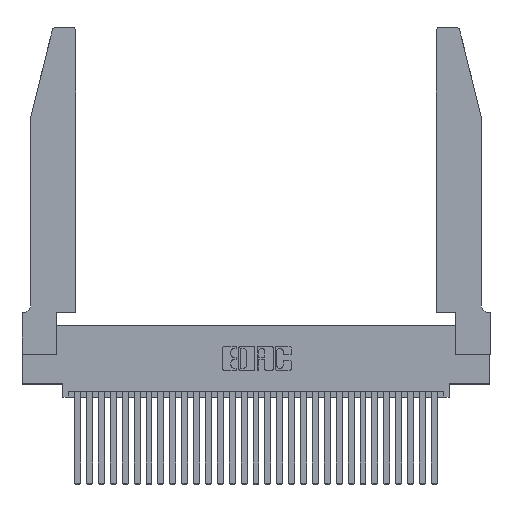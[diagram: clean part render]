
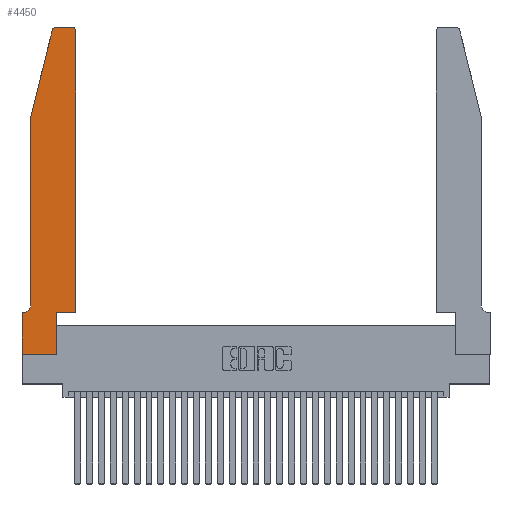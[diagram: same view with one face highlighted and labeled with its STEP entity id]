
A CAD part, top view. The second image highlights one B-rep face of the part: STEP entity #4450.
In plain terms, the highlighted planar face has unit normal (0, 0, 1).
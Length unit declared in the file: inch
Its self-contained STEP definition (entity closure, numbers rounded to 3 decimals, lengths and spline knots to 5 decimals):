
#511 = ORIENTED_EDGE ( 'NONE', *, *, #5564, .T. ) ;
#609 = LINE ( 'NONE', #2005, #8387 ) ;
#863 = VERTEX_POINT ( 'NONE', #15169 ) ;
#949 = VERTEX_POINT ( 'NONE', #22294 ) ;
#1247 = DIRECTION ( 'NONE',  ( 0., 1., 0. ) ) ;
#1689 = EDGE_CURVE ( 'NONE', #27433, #24652, #21861, .T. ) ;
#1990 = VECTOR ( 'NONE', #19626, 39.37008 ) ;
#2004 = ORIENTED_EDGE ( 'NONE', *, *, #20247, .T. ) ;
#2005 = CARTESIAN_POINT ( 'NONE',  ( 0., 0., 0.37 ) ) ;
#2236 = DIRECTION ( 'NONE',  ( 0., 0., -1. ) ) ;
#2530 = EDGE_LOOP ( 'NONE', ( #2004, #16556, #6188, #18421, #3329, #511, #29749, #9568, #21064, #11700, #13305, #5034 ) ) ;
#2979 = CIRCLE ( 'NONE', #29999, 0.03 ) ;
#3178 = LINE ( 'NONE', #10219, #20164 ) ;
#3296 = EDGE_CURVE ( 'NONE', #24652, #29688, #6993, .T. ) ;
#3329 = ORIENTED_EDGE ( 'NONE', *, *, #3296, .T. ) ;
#3477 = CARTESIAN_POINT ( 'NONE',  ( 0.4505, 0.35, 0.37 ) ) ;
#3782 = CARTESIAN_POINT ( 'NONE',  ( 0.284, 2.72, 0.37 ) ) ;
#4260 = CIRCLE ( 'NONE', #22508, 0.03 ) ;
#4450 = ADVANCED_FACE ( 'NONE', ( #7316 ), #19434, .T. ) ;
#4697 = CARTESIAN_POINT ( 'NONE',  ( 0., 0.35, 0.37 ) ) ;
#5034 = ORIENTED_EDGE ( 'NONE', *, *, #11345, .T. ) ;
#5291 = CARTESIAN_POINT ( 'NONE',  ( 0., 0.35, 0.37 ) ) ;
#5395 = CARTESIAN_POINT ( 'NONE',  ( 0.4505, 0.35, 0.37 ) ) ;
#5413 = EDGE_CURVE ( 'NONE', #16458, #863, #609, .T. ) ;
#5564 = EDGE_CURVE ( 'NONE', #29688, #20118, #5778, .T. ) ;
#5778 = LINE ( 'NONE', #12464, #22053 ) ;
#5947 = VERTEX_POINT ( 'NONE', #18750 ) ;
#6188 = ORIENTED_EDGE ( 'NONE', *, *, #13436, .T. ) ;
#6993 = CIRCLE ( 'NONE', #27061, 0.07 ) ;
#7275 = CARTESIAN_POINT ( 'NONE',  ( 0.0755, 2., 0.37 ) ) ;
#7316 = FACE_OUTER_BOUND ( 'NONE', #2530, .T. ) ;
#7475 = VECTOR ( 'NONE', #29697, 39.37008 ) ;
#7598 = CARTESIAN_POINT ( 'NONE',  ( 0.4505, 0.35, 0.37 ) ) ;
#7795 = CARTESIAN_POINT ( 'NONE',  ( 0.2865, 0.35, 0.37 ) ) ;
#8081 = DIRECTION ( 'NONE',  ( 1., 0., 0. ) ) ;
#8289 = CARTESIAN_POINT ( 'NONE',  ( 0.0755, 0.42, 0.37 ) ) ;
#8387 = VECTOR ( 'NONE', #18550, 39.37008 ) ;
#9568 = ORIENTED_EDGE ( 'NONE', *, *, #5413, .T. ) ;
#9693 = VERTEX_POINT ( 'NONE', #22281 ) ;
#10219 = CARTESIAN_POINT ( 'NONE',  ( 0., 0., 0.37 ) ) ;
#10857 = VECTOR ( 'NONE', #1247, 39.37008 ) ;
#11345 = EDGE_CURVE ( 'NONE', #26692, #26193, #4260, .T. ) ;
#11627 = CARTESIAN_POINT ( 'NONE',  ( 0.4205, 2.72, 0.37 ) ) ;
#11700 = ORIENTED_EDGE ( 'NONE', *, *, #16725, .T. ) ;
#12464 = CARTESIAN_POINT ( 'NONE',  ( 0.0755, 0.35, 0.37 ) ) ;
#13305 = ORIENTED_EDGE ( 'NONE', *, *, #16159, .T. ) ;
#13436 = EDGE_CURVE ( 'NONE', #9693, #27433, #21874, .T. ) ;
#13521 = LINE ( 'NONE', #7598, #23506 ) ;
#14630 = DIRECTION ( 'NONE',  ( -1., 0., 0. ) ) ;
#15169 = CARTESIAN_POINT ( 'NONE',  ( 0.2865, 0., 0.37 ) ) ;
#16020 = CARTESIAN_POINT ( 'NONE',  ( 0.4205, 2.75, 0.37 ) ) ;
#16159 = EDGE_CURVE ( 'NONE', #23349, #26692, #13521, .T. ) ;
#16260 = AXIS2_PLACEMENT_3D ( 'NONE', #5291, #24674, #8081 ) ;
#16436 = CARTESIAN_POINT ( 'NONE',  ( 0.0055, 0.35, 0.37 ) ) ;
#16458 = VERTEX_POINT ( 'NONE', #20772 ) ;
#16556 = ORIENTED_EDGE ( 'NONE', *, *, #25343, .T. ) ;
#16725 = EDGE_CURVE ( 'NONE', #5947, #23349, #27804, .T. ) ;
#17133 = LINE ( 'NONE', #7795, #10857 ) ;
#17787 = VECTOR ( 'NONE', #23901, 39.37008 ) ;
#17988 = CARTESIAN_POINT ( 'NONE',  ( 0.0755, 2., 0.37 ) ) ;
#18035 = DIRECTION ( 'NONE',  ( 1., 0., 0. ) ) ;
#18169 = EDGE_CURVE ( 'NONE', #863, #5947, #17133, .T. ) ;
#18421 = ORIENTED_EDGE ( 'NONE', *, *, #1689, .T. ) ;
#18470 = VECTOR ( 'NONE', #26938, 39.37008 ) ;
#18550 = DIRECTION ( 'NONE',  ( 1., 0., 0. ) ) ;
#18750 = CARTESIAN_POINT ( 'NONE',  ( 0.2865, 0.35, 0.37 ) ) ;
#19434 = PLANE ( 'NONE',  #16260 ) ;
#19626 = DIRECTION ( 'NONE',  ( 1., 0., 0. ) ) ;
#19957 = CARTESIAN_POINT ( 'NONE',  ( 0.2605, 2.75, 0.37 ) ) ;
#20022 = CARTESIAN_POINT ( 'NONE',  ( 0.4505, 2.72, 0.37 ) ) ;
#20080 = CARTESIAN_POINT ( 'NONE',  ( 0.0755, 2., 0.37 ) ) ;
#20118 = VERTEX_POINT ( 'NONE', #4697 ) ;
#20164 = VECTOR ( 'NONE', #28895, 39.37008 ) ;
#20247 = EDGE_CURVE ( 'NONE', #26193, #949, #20685, .T. ) ;
#20597 = DIRECTION ( 'NONE',  ( 1., 0., 0. ) ) ;
#20685 = LINE ( 'NONE', #19957, #18470 ) ;
#20772 = CARTESIAN_POINT ( 'NONE',  ( 0., 0., 0.37 ) ) ;
#21064 = ORIENTED_EDGE ( 'NONE', *, *, #18169, .T. ) ;
#21256 = CARTESIAN_POINT ( 'NONE',  ( 0.0055, 0.42, 0.37 ) ) ;
#21444 = EDGE_CURVE ( 'NONE', #20118, #16458, #3178, .T. ) ;
#21861 = LINE ( 'NONE', #7275, #17787 ) ;
#21874 = LINE ( 'NONE', #17988, #7475 ) ;
#22053 = VECTOR ( 'NONE', #14630, 39.37008 ) ;
#22281 = CARTESIAN_POINT ( 'NONE',  ( 0.25487, 2.72718, 0.37 ) ) ;
#22294 = CARTESIAN_POINT ( 'NONE',  ( 0.284, 2.75, 0.37 ) ) ;
#22497 = DIRECTION ( 'NONE',  ( 0., 0., 1. ) ) ;
#22508 = AXIS2_PLACEMENT_3D ( 'NONE', #11627, #27858, #20597 ) ;
#23349 = VERTEX_POINT ( 'NONE', #3477 ) ;
#23506 = VECTOR ( 'NONE', #24354, 39.37008 ) ;
#23901 = DIRECTION ( 'NONE',  ( 0., -1., 0. ) ) ;
#24354 = DIRECTION ( 'NONE',  ( 0., 1., 0. ) ) ;
#24652 = VERTEX_POINT ( 'NONE', #8289 ) ;
#24674 = DIRECTION ( 'NONE',  ( 0., 0., 1. ) ) ;
#25343 = EDGE_CURVE ( 'NONE', #949, #9693, #2979, .T. ) ;
#26193 = VERTEX_POINT ( 'NONE', #16020 ) ;
#26692 = VERTEX_POINT ( 'NONE', #20022 ) ;
#26938 = DIRECTION ( 'NONE',  ( -1., 0., 0. ) ) ;
#27061 = AXIS2_PLACEMENT_3D ( 'NONE', #21256, #2236, #30362 ) ;
#27433 = VERTEX_POINT ( 'NONE', #20080 ) ;
#27804 = LINE ( 'NONE', #5395, #1990 ) ;
#27858 = DIRECTION ( 'NONE',  ( 0., 0., 1. ) ) ;
#28895 = DIRECTION ( 'NONE',  ( 0., -1., 0. ) ) ;
#29688 = VERTEX_POINT ( 'NONE', #16436 ) ;
#29697 = DIRECTION ( 'NONE',  ( -0.239, -0.971, 0. ) ) ;
#29749 = ORIENTED_EDGE ( 'NONE', *, *, #21444, .T. ) ;
#29999 = AXIS2_PLACEMENT_3D ( 'NONE', #3782, #22497, #18035 ) ;
#30362 = DIRECTION ( 'NONE',  ( -1., 0., 0. ) ) ;
